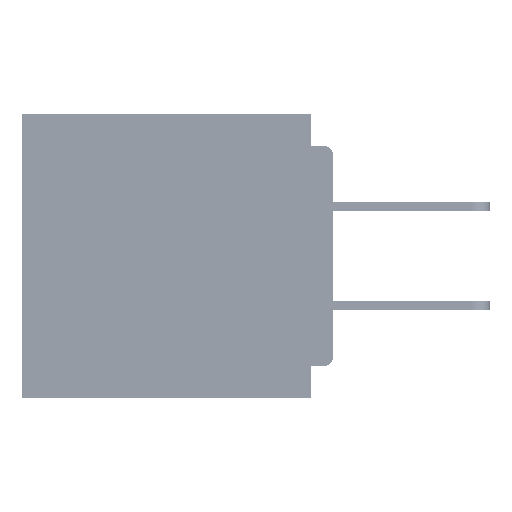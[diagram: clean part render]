
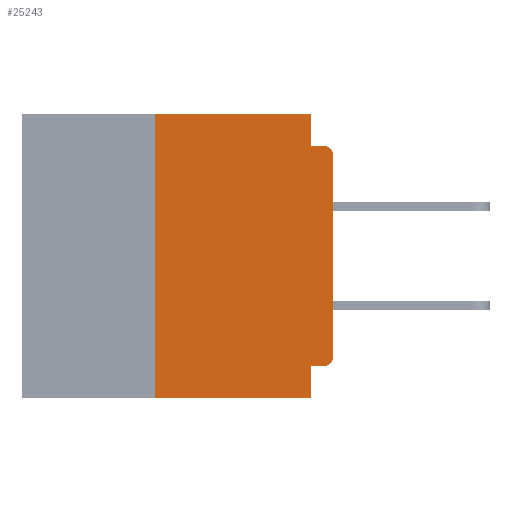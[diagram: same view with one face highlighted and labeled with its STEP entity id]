
A CAD part, left-side view. The second image highlights one B-rep face of the part: STEP entity #25243.
In plain terms, the highlighted planar face has unit normal (-1, 0, 0).
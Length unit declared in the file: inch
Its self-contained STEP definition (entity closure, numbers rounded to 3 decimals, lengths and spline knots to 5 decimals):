
#111 = CARTESIAN_POINT ( 'NONE',  ( 0., 0.031, -0.4 ) ) ;
#644 = CARTESIAN_POINT ( 'NONE',  ( 0., 0., -0.34 ) ) ;
#1761 = DIRECTION ( 'NONE',  ( 0., -1., 0. ) ) ;
#4165 = CARTESIAN_POINT ( 'NONE',  ( 0., 0.031, 0. ) ) ;
#5325 = DIRECTION ( 'NONE',  ( 0., 0., 1. ) ) ;
#5645 = AXIS2_PLACEMENT_3D ( 'NONE', #30006, #61116, #35042 ) ;
#7461 = VERTEX_POINT ( 'NONE', #8090 ) ;
#7578 = VERTEX_POINT ( 'NONE', #8959 ) ;
#7590 = VERTEX_POINT ( 'NONE', #13850 ) ;
#8090 = CARTESIAN_POINT ( 'NONE',  ( 0., 0.015, -0.355 ) ) ;
#8293 = EDGE_CURVE ( 'NONE', #46541, #15516, #32480, .T. ) ;
#8959 = CARTESIAN_POINT ( 'NONE',  ( 0., 0.031, -0.4 ) ) ;
#10137 = VERTEX_POINT ( 'NONE', #644 ) ;
#10831 = VECTOR ( 'NONE', #56351, 39.37008 ) ;
#10920 = CARTESIAN_POINT ( 'NONE',  ( 0., 0.25, 0. ) ) ;
#11972 = CARTESIAN_POINT ( 'NONE',  ( 0., 0.437, 0. ) ) ;
#12326 = ORIENTED_EDGE ( 'NONE', *, *, #39792, .T. ) ;
#12715 = VECTOR ( 'NONE', #39319, 39.37008 ) ;
#13791 = LINE ( 'NONE', #40479, #38831 ) ;
#13850 = CARTESIAN_POINT ( 'NONE',  ( 0., 0.25, -0.4 ) ) ;
#14930 = ORIENTED_EDGE ( 'NONE', *, *, #37724, .F. ) ;
#15275 = CIRCLE ( 'NONE', #21904, 0.015 ) ;
#15516 = VERTEX_POINT ( 'NONE', #27800 ) ;
#17310 = CARTESIAN_POINT ( 'NONE',  ( 0., 0., -0.06 ) ) ;
#17484 = ORIENTED_EDGE ( 'NONE', *, *, #26848, .T. ) ;
#17633 = VECTOR ( 'NONE', #50695, 39.37008 ) ;
#20496 = CARTESIAN_POINT ( 'NONE',  ( 0., 0., -0.045 ) ) ;
#21369 = CARTESIAN_POINT ( 'NONE',  ( 0., 0.437, -0.4 ) ) ;
#21904 = AXIS2_PLACEMENT_3D ( 'NONE', #58711, #28782, #63755 ) ;
#22322 = CARTESIAN_POINT ( 'NONE',  ( 0., 0.031, -0.355 ) ) ;
#22547 = LINE ( 'NONE', #21369, #10831 ) ;
#23190 = EDGE_CURVE ( 'NONE', #7590, #7578, #22547, .T. ) ;
#25243 = ADVANCED_FACE ( 'NONE', ( #40552 ), #58252, .F. ) ;
#26848 = EDGE_CURVE ( 'NONE', #10137, #51486, #13791, .T. ) ;
#27466 = ORIENTED_EDGE ( 'NONE', *, *, #8293, .F. ) ;
#27800 = CARTESIAN_POINT ( 'NONE',  ( 0., 0.015, -0.045 ) ) ;
#28705 = LINE ( 'NONE', #11972, #53789 ) ;
#28782 = DIRECTION ( 'NONE',  ( -1., 0., 0. ) ) ;
#29840 = VERTEX_POINT ( 'NONE', #63075 ) ;
#30006 = CARTESIAN_POINT ( 'NONE',  ( 0., 0.015, -0.34 ) ) ;
#31788 = EDGE_CURVE ( 'NONE', #7590, #39445, #50806, .T. ) ;
#32480 = LINE ( 'NONE', #20496, #17633 ) ;
#32699 = ORIENTED_EDGE ( 'NONE', *, *, #49366, .T. ) ;
#33339 = DIRECTION ( 'NONE',  ( 0., 0., -1. ) ) ;
#35042 = DIRECTION ( 'NONE',  ( 0., 0., -1. ) ) ;
#35447 = CARTESIAN_POINT ( 'NONE',  ( 0., 0.25, -0.4 ) ) ;
#36205 = EDGE_CURVE ( 'NONE', #29840, #46541, #39341, .T. ) ;
#36640 = CARTESIAN_POINT ( 'NONE',  ( 0., 0.031, -0.045 ) ) ;
#37099 = VERTEX_POINT ( 'NONE', #22322 ) ;
#37472 = VECTOR ( 'NONE', #60352, 39.37008 ) ;
#37724 = EDGE_CURVE ( 'NONE', #39445, #29840, #28705, .T. ) ;
#38363 = VECTOR ( 'NONE', #42796, 39.37008 ) ;
#38831 = VECTOR ( 'NONE', #5325, 39.37008 ) ;
#39319 = DIRECTION ( 'NONE',  ( 0., 0., -1. ) ) ;
#39341 = LINE ( 'NONE', #4165, #12715 ) ;
#39445 = VERTEX_POINT ( 'NONE', #10920 ) ;
#39792 = EDGE_CURVE ( 'NONE', #51486, #15516, #15275, .T. ) ;
#39980 = LINE ( 'NONE', #62597, #38363 ) ;
#40076 = ORIENTED_EDGE ( 'NONE', *, *, #23190, .T. ) ;
#40479 = CARTESIAN_POINT ( 'NONE',  ( 0., 0., 0. ) ) ;
#40552 = FACE_OUTER_BOUND ( 'NONE', #45205, .T. ) ;
#41239 = DIRECTION ( 'NONE',  ( 0., 0., -1. ) ) ;
#41819 = ORIENTED_EDGE ( 'NONE', *, *, #56942, .F. ) ;
#42796 = DIRECTION ( 'NONE',  ( 0., 1., 0. ) ) ;
#42859 = AXIS2_PLACEMENT_3D ( 'NONE', #48318, #63300, #33339 ) ;
#43723 = ORIENTED_EDGE ( 'NONE', *, *, #31788, .F. ) ;
#45002 = CIRCLE ( 'NONE', #5645, 0.015 ) ;
#45205 = EDGE_LOOP ( 'NONE', ( #17484, #12326, #27466, #48065, #14930, #43723, #40076, #41819, #53988, #32699 ) ) ;
#46541 = VERTEX_POINT ( 'NONE', #36640 ) ;
#48065 = ORIENTED_EDGE ( 'NONE', *, *, #36205, .F. ) ;
#48318 = CARTESIAN_POINT ( 'NONE',  ( 0., 0.437, 0. ) ) ;
#49366 = EDGE_CURVE ( 'NONE', #7461, #10137, #45002, .T. ) ;
#50695 = DIRECTION ( 'NONE',  ( 0., -1., 0. ) ) ;
#50806 = LINE ( 'NONE', #35447, #37472 ) ;
#51486 = VERTEX_POINT ( 'NONE', #17310 ) ;
#53789 = VECTOR ( 'NONE', #1761, 39.37008 ) ;
#53988 = ORIENTED_EDGE ( 'NONE', *, *, #56631, .F. ) ;
#56351 = DIRECTION ( 'NONE',  ( 0., -1., 0. ) ) ;
#56631 = EDGE_CURVE ( 'NONE', #7461, #37099, #39980, .T. ) ;
#56942 = EDGE_CURVE ( 'NONE', #37099, #7578, #61011, .T. ) ;
#58252 = PLANE ( 'NONE',  #42859 ) ;
#58711 = CARTESIAN_POINT ( 'NONE',  ( 0., 0.015, -0.06 ) ) ;
#59412 = VECTOR ( 'NONE', #41239, 39.37008 ) ;
#60352 = DIRECTION ( 'NONE',  ( 0., 0., 1. ) ) ;
#61011 = LINE ( 'NONE', #111, #59412 ) ;
#61116 = DIRECTION ( 'NONE',  ( -1., 0., 0. ) ) ;
#62597 = CARTESIAN_POINT ( 'NONE',  ( 0., 0., -0.355 ) ) ;
#63075 = CARTESIAN_POINT ( 'NONE',  ( 0., 0.031, 0. ) ) ;
#63300 = DIRECTION ( 'NONE',  ( 1., 0., 0. ) ) ;
#63755 = DIRECTION ( 'NONE',  ( 0., 0., -1. ) ) ;
